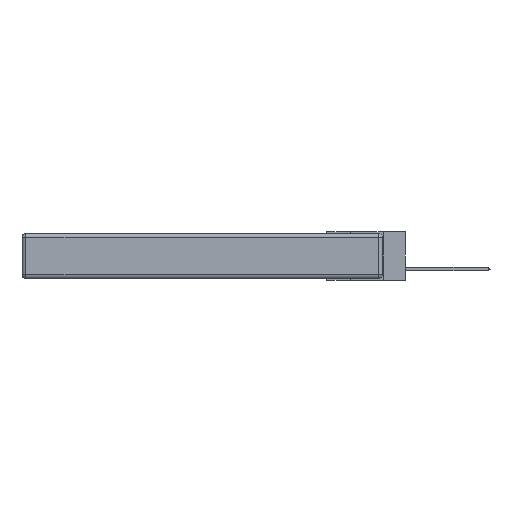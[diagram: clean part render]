
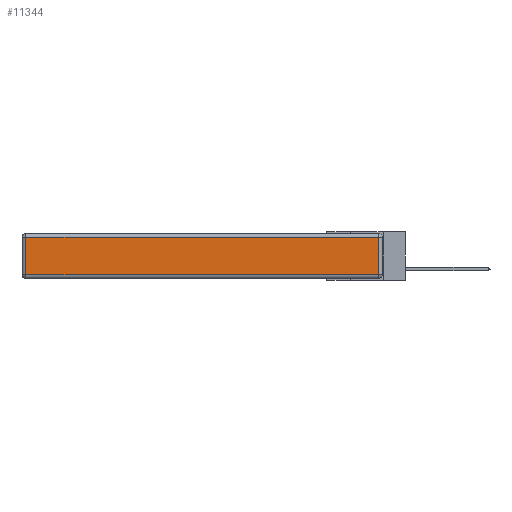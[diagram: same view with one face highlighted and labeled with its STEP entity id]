
A CAD part, left-side view. The second image highlights one B-rep face of the part: STEP entity #11344.
In plain terms, the highlighted planar face has unit normal (-1, 0, 0).
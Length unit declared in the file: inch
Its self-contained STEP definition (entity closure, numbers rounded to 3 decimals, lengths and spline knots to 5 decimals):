
#227 = CARTESIAN_POINT ( 'NONE',  ( 0., 0.03, -0.313 ) ) ;
#865 = CARTESIAN_POINT ( 'NONE',  ( 0., 0.03, -0.03 ) ) ;
#959 = DIRECTION ( 'NONE',  ( 0., -1., 0. ) ) ;
#1424 = VERTEX_POINT ( 'NONE', #865 ) ;
#1464 = DIRECTION ( 'NONE',  ( 0., 1., 0. ) ) ;
#2274 = LINE ( 'NONE', #2774, #9328 ) ;
#2462 = VERTEX_POINT ( 'NONE', #227 ) ;
#2774 = CARTESIAN_POINT ( 'NONE',  ( 0., 0.03, -0.343 ) ) ;
#3915 = CARTESIAN_POINT ( 'NONE',  ( 0., 2.72, -0.313 ) ) ;
#3946 = CARTESIAN_POINT ( 'NONE',  ( 0., 0., -0.313 ) ) ;
#4030 = FACE_OUTER_BOUND ( 'NONE', #7004, .T. ) ;
#4349 = LINE ( 'NONE', #11663, #9799 ) ;
#4825 = ORIENTED_EDGE ( 'NONE', *, *, #9933, .T. ) ;
#4926 = CARTESIAN_POINT ( 'NONE',  ( 0., 0., -0.343 ) ) ;
#5049 = DIRECTION ( 'NONE',  ( -1., 0., 0. ) ) ;
#6169 = AXIS2_PLACEMENT_3D ( 'NONE', #4926, #5049, #8079 ) ;
#6354 = VERTEX_POINT ( 'NONE', #9631 ) ;
#7004 = EDGE_LOOP ( 'NONE', ( #4825, #7301, #12386, #11068 ) ) ;
#7301 = ORIENTED_EDGE ( 'NONE', *, *, #11116, .T. ) ;
#7993 = PLANE ( 'NONE',  #6169 ) ;
#8079 = DIRECTION ( 'NONE',  ( 0., 0., 1. ) ) ;
#8131 = EDGE_CURVE ( 'NONE', #1424, #6354, #4349, .T. ) ;
#8854 = LINE ( 'NONE', #3946, #12873 ) ;
#9292 = VECTOR ( 'NONE', #10778, 39.37008 ) ;
#9328 = VECTOR ( 'NONE', #11210, 39.37008 ) ;
#9400 = VERTEX_POINT ( 'NONE', #3915 ) ;
#9631 = CARTESIAN_POINT ( 'NONE',  ( 0., 2.72, -0.03 ) ) ;
#9799 = VECTOR ( 'NONE', #1464, 39.37008 ) ;
#9933 = EDGE_CURVE ( 'NONE', #9400, #2462, #8854, .T. ) ;
#10778 = DIRECTION ( 'NONE',  ( 0., 0., -1. ) ) ;
#11068 = ORIENTED_EDGE ( 'NONE', *, *, #12492, .T. ) ;
#11116 = EDGE_CURVE ( 'NONE', #2462, #1424, #2274, .T. ) ;
#11210 = DIRECTION ( 'NONE',  ( 0., 0., 1. ) ) ;
#11344 = ADVANCED_FACE ( 'NONE', ( #4030 ), #7993, .T. ) ;
#11663 = CARTESIAN_POINT ( 'NONE',  ( 0., 2.75, -0.03 ) ) ;
#12386 = ORIENTED_EDGE ( 'NONE', *, *, #8131, .T. ) ;
#12492 = EDGE_CURVE ( 'NONE', #6354, #9400, #13131, .T. ) ;
#12606 = CARTESIAN_POINT ( 'NONE',  ( 0., 2.72, -0.343 ) ) ;
#12873 = VECTOR ( 'NONE', #959, 39.37008 ) ;
#13131 = LINE ( 'NONE', #12606, #9292 ) ;
